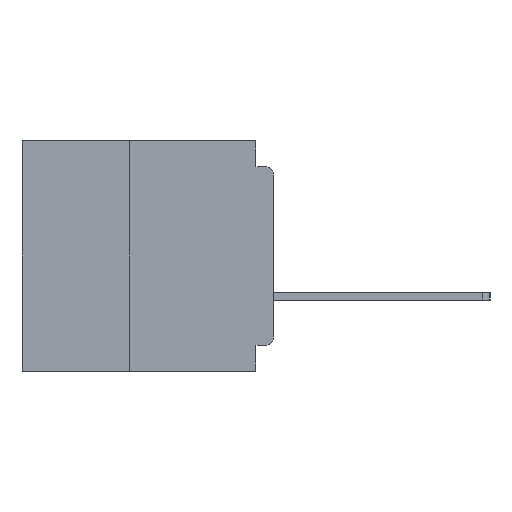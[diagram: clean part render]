
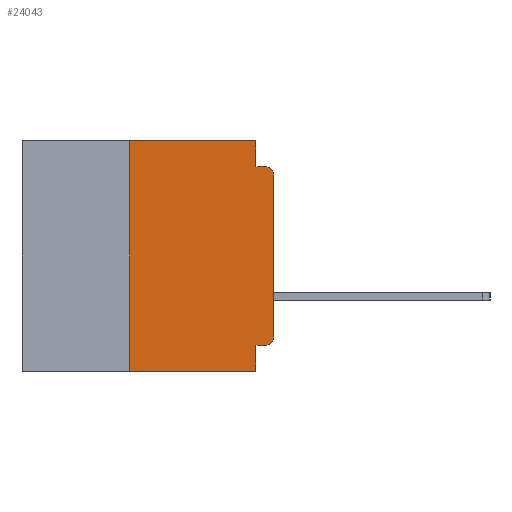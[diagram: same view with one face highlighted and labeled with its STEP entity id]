
A CAD part, left-side view. The second image highlights one B-rep face of the part: STEP entity #24043.
In plain terms, the highlighted planar face has unit normal (-1, 0, 0).
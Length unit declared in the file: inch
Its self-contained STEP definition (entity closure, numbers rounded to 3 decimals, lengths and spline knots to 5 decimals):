
#679 = VERTEX_POINT ( 'NONE', #33468 ) ;
#937 = EDGE_CURVE ( 'NONE', #45060, #38161, #28976, .T. ) ;
#1018 = VERTEX_POINT ( 'NONE', #6420 ) ;
#1279 = DIRECTION ( 'NONE',  ( -1., 0., 0. ) ) ;
#1354 = DIRECTION ( 'NONE',  ( 0., 0., -1. ) ) ;
#1848 = FACE_OUTER_BOUND ( 'NONE', #28737, .T. ) ;
#1929 = ORIENTED_EDGE ( 'NONE', *, *, #35971, .F. ) ;
#3770 = CARTESIAN_POINT ( 'NONE',  ( 0., 0.25, -0.4 ) ) ;
#4136 = LINE ( 'NONE', #6934, #47434 ) ;
#4559 = CARTESIAN_POINT ( 'NONE',  ( 0., 0.031, 0. ) ) ;
#4701 = CARTESIAN_POINT ( 'NONE',  ( 0., 0., -0.355 ) ) ;
#4793 = DIRECTION ( 'NONE',  ( 0., 0., -1. ) ) ;
#5479 = CARTESIAN_POINT ( 'NONE',  ( 0., 0., -0.34 ) ) ;
#6420 = CARTESIAN_POINT ( 'NONE',  ( 0., 0.25, 0. ) ) ;
#6934 = CARTESIAN_POINT ( 'NONE',  ( 0., 0., -0.045 ) ) ;
#7024 = LINE ( 'NONE', #4701, #39569 ) ;
#8398 = CARTESIAN_POINT ( 'NONE',  ( 0., 0.015, -0.045 ) ) ;
#8842 = CARTESIAN_POINT ( 'NONE',  ( 0., 0.437, -0.4 ) ) ;
#8932 = CARTESIAN_POINT ( 'NONE',  ( 0., 0.25, -0.4 ) ) ;
#9379 = EDGE_CURVE ( 'NONE', #17879, #21066, #12141, .T. ) ;
#10092 = AXIS2_PLACEMENT_3D ( 'NONE', #50121, #25975, #1354 ) ;
#11530 = CARTESIAN_POINT ( 'NONE',  ( 0., 0.031, -0.4 ) ) ;
#11860 = DIRECTION ( 'NONE',  ( 0., 0., 1. ) ) ;
#12141 = CIRCLE ( 'NONE', #33874, 0.015 ) ;
#12372 = VERTEX_POINT ( 'NONE', #32263 ) ;
#12396 = PLANE ( 'NONE',  #43840 ) ;
#12729 = DIRECTION ( 'NONE',  ( 1., 0., 0. ) ) ;
#13584 = EDGE_CURVE ( 'NONE', #26872, #43469, #39243, .T. ) ;
#16032 = CARTESIAN_POINT ( 'NONE',  ( 0., 0., -0.06 ) ) ;
#16813 = CARTESIAN_POINT ( 'NONE',  ( 0., 0.031, 0. ) ) ;
#17152 = CIRCLE ( 'NONE', #10092, 0.015 ) ;
#17700 = ORIENTED_EDGE ( 'NONE', *, *, #13584, .T. ) ;
#17879 = VERTEX_POINT ( 'NONE', #16032 ) ;
#19037 = LINE ( 'NONE', #49720, #28620 ) ;
#19137 = VECTOR ( 'NONE', #11860, 39.37008 ) ;
#19320 = LINE ( 'NONE', #11530, #30149 ) ;
#19909 = CARTESIAN_POINT ( 'NONE',  ( 0., 0.031, -0.4 ) ) ;
#21066 = VERTEX_POINT ( 'NONE', #8398 ) ;
#21282 = ORIENTED_EDGE ( 'NONE', *, *, #36034, .F. ) ;
#24043 = ADVANCED_FACE ( 'NONE', ( #1848 ), #12396, .F. ) ;
#24516 = ORIENTED_EDGE ( 'NONE', *, *, #52319, .F. ) ;
#25891 = CARTESIAN_POINT ( 'NONE',  ( 0., 0.015, -0.06 ) ) ;
#25975 = DIRECTION ( 'NONE',  ( -1., 0., 0. ) ) ;
#26872 = VERTEX_POINT ( 'NONE', #8932 ) ;
#27089 = ORIENTED_EDGE ( 'NONE', *, *, #50534, .T. ) ;
#28476 = VECTOR ( 'NONE', #37377, 39.37008 ) ;
#28620 = VECTOR ( 'NONE', #41808, 39.37008 ) ;
#28737 = EDGE_LOOP ( 'NONE', ( #27089, #37552, #24516, #45314, #32766, #21282, #17700, #1929, #35178, #37531 ) ) ;
#28882 = VECTOR ( 'NONE', #32452, 39.37008 ) ;
#28976 = LINE ( 'NONE', #4559, #49161 ) ;
#29815 = EDGE_CURVE ( 'NONE', #679, #12372, #7024, .T. ) ;
#29962 = DIRECTION ( 'NONE',  ( 0., 0., -1. ) ) ;
#29971 = LINE ( 'NONE', #36272, #19137 ) ;
#30149 = VECTOR ( 'NONE', #31931, 39.37008 ) ;
#31159 = VERTEX_POINT ( 'NONE', #5479 ) ;
#31931 = DIRECTION ( 'NONE',  ( 0., 0., -1. ) ) ;
#32263 = CARTESIAN_POINT ( 'NONE',  ( 0., 0.031, -0.355 ) ) ;
#32452 = DIRECTION ( 'NONE',  ( 0., 0., 1. ) ) ;
#32766 = ORIENTED_EDGE ( 'NONE', *, *, #51451, .F. ) ;
#33328 = DIRECTION ( 'NONE',  ( 0., 1., 0. ) ) ;
#33468 = CARTESIAN_POINT ( 'NONE',  ( 0., 0.015, -0.355 ) ) ;
#33874 = AXIS2_PLACEMENT_3D ( 'NONE', #25891, #1279, #29962 ) ;
#35178 = ORIENTED_EDGE ( 'NONE', *, *, #29815, .F. ) ;
#35487 = DIRECTION ( 'NONE',  ( 0., -1., 0. ) ) ;
#35971 = EDGE_CURVE ( 'NONE', #12372, #43469, #19320, .T. ) ;
#36034 = EDGE_CURVE ( 'NONE', #26872, #1018, #47822, .T. ) ;
#36272 = CARTESIAN_POINT ( 'NONE',  ( 0., 0., 0. ) ) ;
#37159 = CARTESIAN_POINT ( 'NONE',  ( 0., 0.437, 0. ) ) ;
#37377 = DIRECTION ( 'NONE',  ( 0., -1., 0. ) ) ;
#37531 = ORIENTED_EDGE ( 'NONE', *, *, #50824, .T. ) ;
#37552 = ORIENTED_EDGE ( 'NONE', *, *, #9379, .T. ) ;
#38161 = VERTEX_POINT ( 'NONE', #47756 ) ;
#39243 = LINE ( 'NONE', #8842, #28476 ) ;
#39569 = VECTOR ( 'NONE', #33328, 39.37008 ) ;
#41220 = DIRECTION ( 'NONE',  ( 0., 0., -1. ) ) ;
#41808 = DIRECTION ( 'NONE',  ( 0., -1., 0. ) ) ;
#43469 = VERTEX_POINT ( 'NONE', #19909 ) ;
#43840 = AXIS2_PLACEMENT_3D ( 'NONE', #37159, #12729, #41220 ) ;
#45060 = VERTEX_POINT ( 'NONE', #16813 ) ;
#45314 = ORIENTED_EDGE ( 'NONE', *, *, #937, .F. ) ;
#47434 = VECTOR ( 'NONE', #35487, 39.37008 ) ;
#47756 = CARTESIAN_POINT ( 'NONE',  ( 0., 0.031, -0.045 ) ) ;
#47822 = LINE ( 'NONE', #3770, #28882 ) ;
#49161 = VECTOR ( 'NONE', #4793, 39.37008 ) ;
#49720 = CARTESIAN_POINT ( 'NONE',  ( 0., 0.437, 0. ) ) ;
#50121 = CARTESIAN_POINT ( 'NONE',  ( 0., 0.015, -0.34 ) ) ;
#50534 = EDGE_CURVE ( 'NONE', #31159, #17879, #29971, .T. ) ;
#50824 = EDGE_CURVE ( 'NONE', #679, #31159, #17152, .T. ) ;
#51451 = EDGE_CURVE ( 'NONE', #1018, #45060, #19037, .T. ) ;
#52319 = EDGE_CURVE ( 'NONE', #38161, #21066, #4136, .T. ) ;
